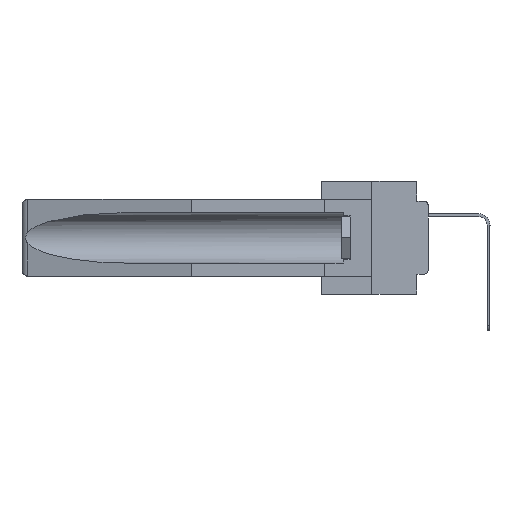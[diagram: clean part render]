
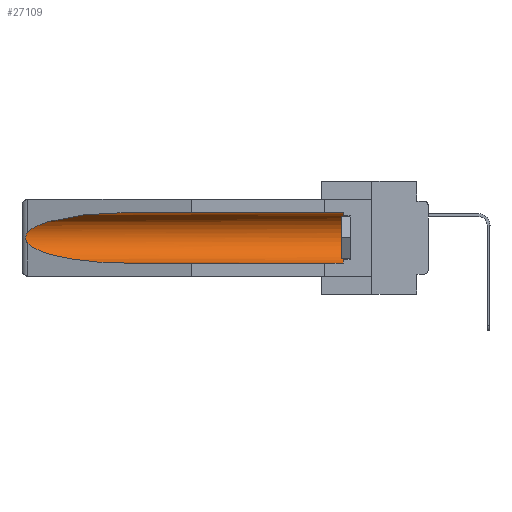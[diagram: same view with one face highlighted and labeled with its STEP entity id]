
A CAD part, left-side view. The second image highlights one B-rep face of the part: STEP entity #27109.
In plain terms, the highlighted cylindrical face has radius 2.857 mm (diameter 5.715 mm), a partial arc.
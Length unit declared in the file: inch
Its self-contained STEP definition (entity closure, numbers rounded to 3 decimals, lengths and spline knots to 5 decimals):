
#472 = CARTESIAN_POINT ( 'NONE',  ( 0.155, 1.07973, -0.059 ) ) ;
#1111 = CARTESIAN_POINT ( 'NONE',  ( 0.155, 1.07973, -0.284 ) ) ;
#1705 = CARTESIAN_POINT ( 'NONE',  ( 0.26654, 1.53092, -0.15636 ) ) ;
#1821 = CARTESIAN_POINT ( 'NONE',  ( 0.26537, 1.52718, -0.14972 ) ) ;
#2013 = ORIENTED_EDGE ( 'NONE', *, *, #26885, .T. ) ;
#2073 = B_SPLINE_CURVE_WITH_KNOTS ( 'NONE', 3,
 ( #1821, #34621, #1705, #10023, #23812, #34851, #4476, #26334, #9905, #31968 ),
 .UNSPECIFIED., .F., .F.,
 ( 4, 2, 2, 2, 4 ),
 ( 0., 0.00029, 0.00058, 0.00087, 0.00117 ),
 .UNSPECIFIED. ) ;
#2560 = ORIENTED_EDGE ( 'NONE', *, *, #32289, .T. ) ;
#3276 = CARTESIAN_POINT ( 'NONE',  ( 0.26537, 1.52718, -0.14972 ) ) ;
#3801 = VECTOR ( 'NONE', #21544, 39.37008 ) ;
#4476 = CARTESIAN_POINT ( 'NONE',  ( 0.2673, 1.53269, -0.17917 ) ) ;
#4927 = CARTESIAN_POINT ( 'NONE',  ( 0.26537, 1.52718, -0.14972 ) ) ;
#6293 = CARTESIAN_POINT ( 'NONE',  ( 0.26537, 1.52718, -0.19328 ) ) ;
#7169 = CARTESIAN_POINT ( 'NONE',  ( 0.155, 1.07973, -0.059 ) ) ;
#7470 = CIRCLE ( 'NONE', #13558, 0.1125 ) ;
#7998 = VECTOR ( 'NONE', #32834, 39.37008 ) ;
#9064 = EDGE_CURVE ( 'NONE', #21227, #16915, #17568, .T. ) ;
#9632 = ORIENTED_EDGE ( 'NONE', *, *, #14956, .T. ) ;
#9905 = CARTESIAN_POINT ( 'NONE',  ( 0.26597, 1.5296, -0.19026 ) ) ;
#10023 = CARTESIAN_POINT ( 'NONE',  ( 0.2673, 1.5327, -0.16383 ) ) ;
#10154 = LINE ( 'NONE', #16403, #7998 ) ;
#11036 = CARTESIAN_POINT ( 'NONE',  ( 0.155, 0.126, -0.1715 ) ) ;
#12291 = ORIENTED_EDGE ( 'NONE', *, *, #9064, .F. ) ;
#12826 = CARTESIAN_POINT ( 'NONE',  ( 0.155, -0.30754, -0.1715 ) ) ;
#13069 = DIRECTION ( 'NONE',  ( 0., 1., 0. ) ) ;
#13072 = VERTEX_POINT ( 'NONE', #4927 ) ;
#13558 = AXIS2_PLACEMENT_3D ( 'NONE', #11036, #13784, #30586 ) ;
#13784 = DIRECTION ( 'NONE',  ( 0., -1., 0. ) ) ;
#14698 = CARTESIAN_POINT ( 'NONE',  ( 0.25451, 1.48313, -0.24835 ) ) ;
#14956 = EDGE_CURVE ( 'NONE', #20450, #33021, #10154, .T. ) ;
#15597 = DIRECTION ( 'NONE',  ( 0., 0., 1. ) ) ;
#15895 = CARTESIAN_POINT ( 'NONE',  ( 0.155, 0.126, -0.059 ) ) ;
#16101 = EDGE_CURVE ( 'NONE', #21227, #20450, #7470, .T. ) ;
#16403 = CARTESIAN_POINT ( 'NONE',  ( 0.155, -0.30754, -0.059 ) ) ;
#16801 =( BOUNDED_CURVE ( )  B_SPLINE_CURVE ( 3, ( #472, #28346, #19720, #3276 ),
 .UNSPECIFIED., .F., .F. ) 
 B_SPLINE_CURVE_WITH_KNOTS ( ( 4, 4 ),
 ( 4.71239, 6.08839 ),
 .UNSPECIFIED. ) 
 CURVE ( )  GEOMETRIC_REPRESENTATION_ITEM ( )  RATIONAL_B_SPLINE_CURVE ( ( 1., 0.848, 0.848, 1. ) ) 
 REPRESENTATION_ITEM ( '' )  );
#16915 = VERTEX_POINT ( 'NONE', #28363 ) ;
#17568 = LINE ( 'NONE', #19129, #3801 ) ;
#18385 = ORIENTED_EDGE ( 'NONE', *, *, #33607, .T. ) ;
#19129 = CARTESIAN_POINT ( 'NONE',  ( 0.155, -0.30754, -0.284 ) ) ;
#19720 = CARTESIAN_POINT ( 'NONE',  ( 0.25451, 1.48313, -0.09465 ) ) ;
#20450 = VERTEX_POINT ( 'NONE', #15895 ) ;
#21227 = VERTEX_POINT ( 'NONE', #21863 ) ;
#21544 = DIRECTION ( 'NONE',  ( 0., 1., 0. ) ) ;
#21863 = CARTESIAN_POINT ( 'NONE',  ( 0.155, 0.126, -0.284 ) ) ;
#23094 = ORIENTED_EDGE ( 'NONE', *, *, #16101, .T. ) ;
#23162 = VERTEX_POINT ( 'NONE', #23274 ) ;
#23274 = CARTESIAN_POINT ( 'NONE',  ( 0.26537, 1.52718, -0.19328 ) ) ;
#23812 = CARTESIAN_POINT ( 'NONE',  ( 0.2675, 1.53308, -0.16763 ) ) ;
#25823 = EDGE_LOOP ( 'NONE', ( #2560, #2013, #18385, #12291, #23094, #9632 ) ) ;
#26334 = CARTESIAN_POINT ( 'NONE',  ( 0.26655, 1.53094, -0.18657 ) ) ;
#26885 = EDGE_CURVE ( 'NONE', #13072, #23162, #2073, .T. ) ;
#27109 = ADVANCED_FACE ( 'NONE', ( #28943 ), #31544, .F. ) ;
#27159 = AXIS2_PLACEMENT_3D ( 'NONE', #12826, #13069, #15597 ) ;
#28146 = CARTESIAN_POINT ( 'NONE',  ( 0.21114, 1.30732, -0.284 ) ) ;
#28346 = CARTESIAN_POINT ( 'NONE',  ( 0.21114, 1.30732, -0.059 ) ) ;
#28363 = CARTESIAN_POINT ( 'NONE',  ( 0.155, 1.07973, -0.284 ) ) ;
#28943 = FACE_OUTER_BOUND ( 'NONE', #25823, .T. ) ;
#30586 = DIRECTION ( 'NONE',  ( 0., 0., 1. ) ) ;
#31122 =( BOUNDED_CURVE ( )  B_SPLINE_CURVE ( 3, ( #6293, #14698, #28146, #1111 ),
 .UNSPECIFIED., .F., .F. ) 
 B_SPLINE_CURVE_WITH_KNOTS ( ( 4, 4 ),
 ( 0.1948, 1.5708 ),
 .UNSPECIFIED. ) 
 CURVE ( )  GEOMETRIC_REPRESENTATION_ITEM ( )  RATIONAL_B_SPLINE_CURVE ( ( 1., 0.848, 0.848, 1. ) ) 
 REPRESENTATION_ITEM ( '' )  );
#31544 = CYLINDRICAL_SURFACE ( 'NONE', #27159, 0.1125 ) ;
#31968 = CARTESIAN_POINT ( 'NONE',  ( 0.26537, 1.52718, -0.19328 ) ) ;
#32289 = EDGE_CURVE ( 'NONE', #33021, #13072, #16801, .T. ) ;
#32834 = DIRECTION ( 'NONE',  ( 0., 1., 0. ) ) ;
#33021 = VERTEX_POINT ( 'NONE', #7169 ) ;
#33607 = EDGE_CURVE ( 'NONE', #23162, #16915, #31122, .T. ) ;
#34621 = CARTESIAN_POINT ( 'NONE',  ( 0.26597, 1.52961, -0.15275 ) ) ;
#34851 = CARTESIAN_POINT ( 'NONE',  ( 0.2675, 1.53308, -0.17534 ) ) ;
